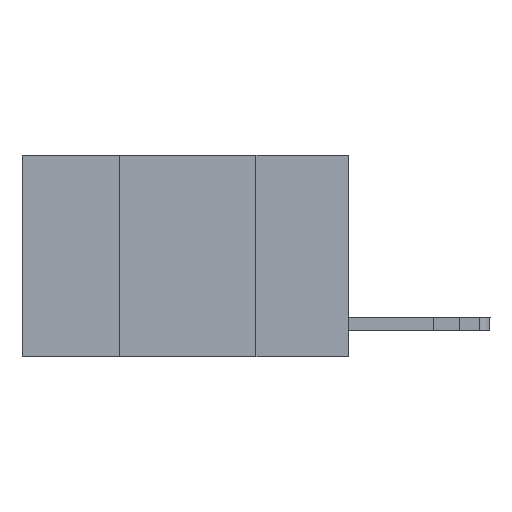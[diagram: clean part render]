
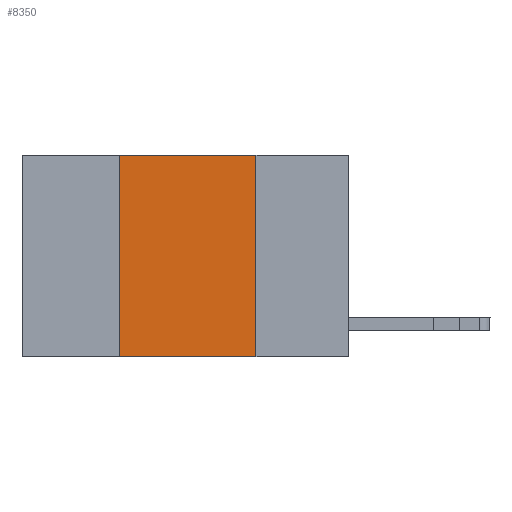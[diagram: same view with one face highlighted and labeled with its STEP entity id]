
A CAD part, left-side view. The second image highlights one B-rep face of the part: STEP entity #8350.
In plain terms, the highlighted planar face has unit normal (-1, 0, 0).
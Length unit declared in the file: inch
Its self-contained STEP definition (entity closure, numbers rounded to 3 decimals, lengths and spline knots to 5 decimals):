
#624 = DIRECTION ( 'NONE',  ( 0., 0., -1. ) ) ;
#1353 = CARTESIAN_POINT ( 'NONE',  ( 0., 0.42, 0. ) ) ;
#1655 = DIRECTION ( 'NONE',  ( 0., 0., 1. ) ) ;
#2910 = VECTOR ( 'NONE', #1655, 39.37008 ) ;
#4675 = DIRECTION ( 'NONE',  ( 0., -1., 0. ) ) ;
#8054 = VERTEX_POINT ( 'NONE', #15539 ) ;
#8350 = ADVANCED_FACE ( 'NONE', ( #14308 ), #14508, .F. ) ;
#8369 = EDGE_CURVE ( 'NONE', #14761, #8054, #15530, .T. ) ;
#8548 = ORIENTED_EDGE ( 'NONE', *, *, #8369, .T. ) ;
#8984 = VECTOR ( 'NONE', #4675, 39.37008 ) ;
#9305 = CARTESIAN_POINT ( 'NONE',  ( 0., 0.17, 0. ) ) ;
#9696 = EDGE_CURVE ( 'NONE', #14761, #23435, #18242, .T. ) ;
#11356 = DIRECTION ( 'NONE',  ( 0., -1., 0. ) ) ;
#12414 = VECTOR ( 'NONE', #25003, 39.37008 ) ;
#12694 = DIRECTION ( 'NONE',  ( 1., 0., 0. ) ) ;
#13231 = ORIENTED_EDGE ( 'NONE', *, *, #9696, .F. ) ;
#13703 = CARTESIAN_POINT ( 'NONE',  ( 0., 0.42, 0. ) ) ;
#13716 = EDGE_CURVE ( 'NONE', #24231, #8054, #22813, .T. ) ;
#14308 = FACE_OUTER_BOUND ( 'NONE', #16593, .T. ) ;
#14508 = PLANE ( 'NONE',  #22292 ) ;
#14677 = CARTESIAN_POINT ( 'NONE',  ( 0., 0.6, -0.37 ) ) ;
#14761 = VERTEX_POINT ( 'NONE', #18875 ) ;
#14881 = EDGE_CURVE ( 'NONE', #23435, #24231, #17917, .T. ) ;
#15530 = LINE ( 'NONE', #14677, #8984 ) ;
#15539 = CARTESIAN_POINT ( 'NONE',  ( 0., 0.17, -0.37 ) ) ;
#15682 = ORIENTED_EDGE ( 'NONE', *, *, #13716, .F. ) ;
#16593 = EDGE_LOOP ( 'NONE', ( #15682, #21509, #13231, #8548 ) ) ;
#17917 = LINE ( 'NONE', #21162, #21245 ) ;
#18242 = LINE ( 'NONE', #13703, #2910 ) ;
#18875 = CARTESIAN_POINT ( 'NONE',  ( 0., 0.42, -0.37 ) ) ;
#21162 = CARTESIAN_POINT ( 'NONE',  ( 0., 0.6, 0. ) ) ;
#21245 = VECTOR ( 'NONE', #11356, 39.37008 ) ;
#21509 = ORIENTED_EDGE ( 'NONE', *, *, #14881, .F. ) ;
#22292 = AXIS2_PLACEMENT_3D ( 'NONE', #24380, #12694, #624 ) ;
#22813 = LINE ( 'NONE', #9305, #12414 ) ;
#23435 = VERTEX_POINT ( 'NONE', #1353 ) ;
#24231 = VERTEX_POINT ( 'NONE', #25662 ) ;
#24380 = CARTESIAN_POINT ( 'NONE',  ( 0., 0.6, 0. ) ) ;
#25003 = DIRECTION ( 'NONE',  ( 0., 0., -1. ) ) ;
#25662 = CARTESIAN_POINT ( 'NONE',  ( 0., 0.17, 0. ) ) ;
